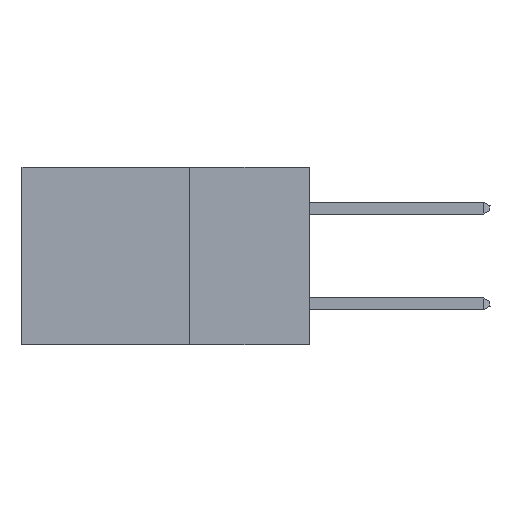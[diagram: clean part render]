
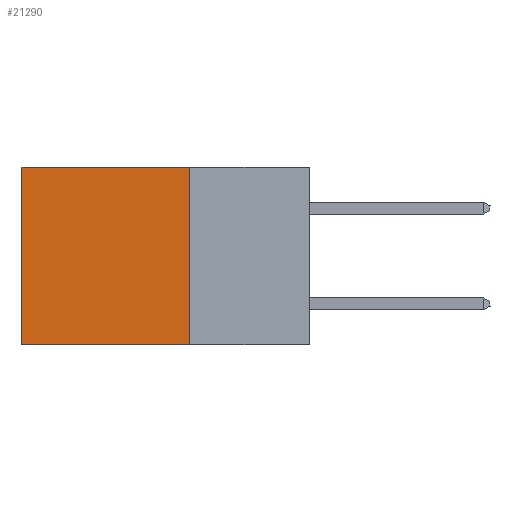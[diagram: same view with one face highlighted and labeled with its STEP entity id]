
A CAD part, left-side view. The second image highlights one B-rep face of the part: STEP entity #21290.
In plain terms, the highlighted planar face has unit normal (-1, 0, 0).
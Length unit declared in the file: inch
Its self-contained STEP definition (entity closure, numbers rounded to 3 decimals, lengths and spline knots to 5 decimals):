
#652 = LINE ( 'NONE', #3063, #28470 ) ;
#1341 = VECTOR ( 'NONE', #4783, 39.37008 ) ;
#1448 = CARTESIAN_POINT ( 'NONE',  ( 0.2875, 0.6, 0. ) ) ;
#2965 = DIRECTION ( 'NONE',  ( 0., 0., -1. ) ) ;
#3063 = CARTESIAN_POINT ( 'NONE',  ( 0.2875, 0.25, 0. ) ) ;
#3085 = ORIENTED_EDGE ( 'NONE', *, *, #24845, .T. ) ;
#3475 = DIRECTION ( 'NONE',  ( 0., 1., 0. ) ) ;
#4206 = DIRECTION ( 'NONE',  ( 1., 0., 0. ) ) ;
#4783 = DIRECTION ( 'NONE',  ( 0., 1., 0. ) ) ;
#9763 = VERTEX_POINT ( 'NONE', #25891 ) ;
#9836 = EDGE_CURVE ( 'NONE', #24361, #17907, #652, .T. ) ;
#12864 = CARTESIAN_POINT ( 'NONE',  ( 0.2875, 0.25, -0.37 ) ) ;
#13008 = ORIENTED_EDGE ( 'NONE', *, *, #9836, .F. ) ;
#13164 = CARTESIAN_POINT ( 'NONE',  ( 0.2875, 0.25, -0.37 ) ) ;
#13454 = LINE ( 'NONE', #13164, #23354 ) ;
#14142 = FACE_OUTER_BOUND ( 'NONE', #22733, .T. ) ;
#14182 = PLANE ( 'NONE',  #28486 ) ;
#14914 = CARTESIAN_POINT ( 'NONE',  ( 0.2875, 0.25, 0. ) ) ;
#15876 = VECTOR ( 'NONE', #2965, 39.37008 ) ;
#16737 = CARTESIAN_POINT ( 'NONE',  ( 0.2875, 0.25, 0. ) ) ;
#17907 = VERTEX_POINT ( 'NONE', #12864 ) ;
#19151 = EDGE_CURVE ( 'NONE', #17907, #9763, #13454, .T. ) ;
#21184 = ORIENTED_EDGE ( 'NONE', *, *, #19151, .F. ) ;
#21290 = ADVANCED_FACE ( 'NONE', ( #14142 ), #14182, .F. ) ;
#21400 = LINE ( 'NONE', #22816, #15876 ) ;
#21906 = DIRECTION ( 'NONE',  ( 0., 0., -1. ) ) ;
#22144 = VERTEX_POINT ( 'NONE', #1448 ) ;
#22733 = EDGE_LOOP ( 'NONE', ( #31337, #21184, #13008, #3085 ) ) ;
#22816 = CARTESIAN_POINT ( 'NONE',  ( 0.2875, 0.6, 0. ) ) ;
#23125 = CARTESIAN_POINT ( 'NONE',  ( 0.2875, 0.25, 0. ) ) ;
#23354 = VECTOR ( 'NONE', #3475, 39.37008 ) ;
#24361 = VERTEX_POINT ( 'NONE', #23125 ) ;
#24845 = EDGE_CURVE ( 'NONE', #24361, #22144, #27943, .T. ) ;
#25666 = DIRECTION ( 'NONE',  ( 0., 0., -1. ) ) ;
#25891 = CARTESIAN_POINT ( 'NONE',  ( 0.2875, 0.6, -0.37 ) ) ;
#27943 = LINE ( 'NONE', #14914, #1341 ) ;
#28470 = VECTOR ( 'NONE', #25666, 39.37008 ) ;
#28486 = AXIS2_PLACEMENT_3D ( 'NONE', #16737, #4206, #21906 ) ;
#28836 = EDGE_CURVE ( 'NONE', #22144, #9763, #21400, .T. ) ;
#31337 = ORIENTED_EDGE ( 'NONE', *, *, #28836, .T. ) ;
